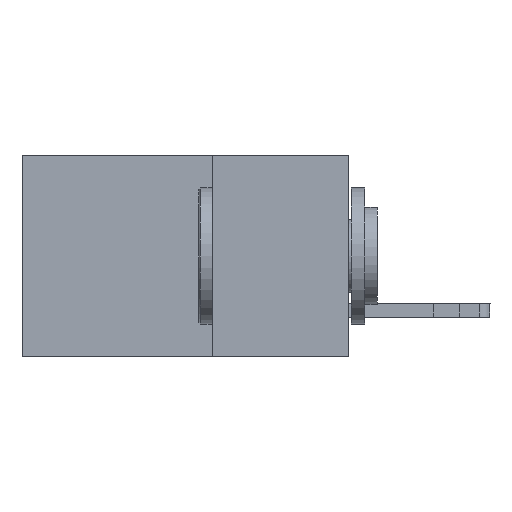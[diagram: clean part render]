
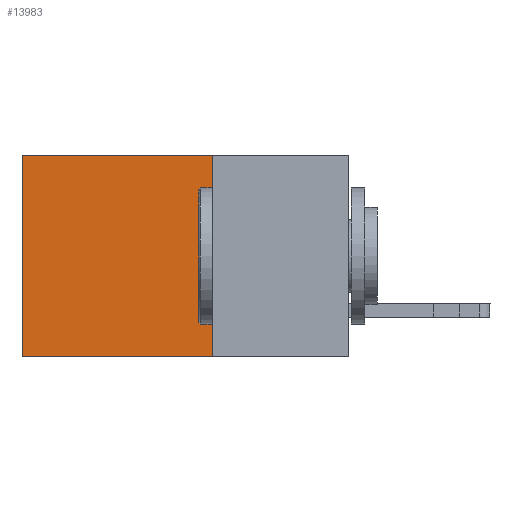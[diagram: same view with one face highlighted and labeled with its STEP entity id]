
A CAD part, left-side view. The second image highlights one B-rep face of the part: STEP entity #13983.
In plain terms, the highlighted planar face has unit normal (-1, 0, 0).
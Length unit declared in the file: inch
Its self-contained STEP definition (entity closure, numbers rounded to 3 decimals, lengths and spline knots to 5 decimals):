
#703 = LINE ( 'NONE', #4443, #17010 ) ;
#2767 = CARTESIAN_POINT ( 'NONE',  ( 0.2615, 0.6, -0.37 ) ) ;
#2885 = CARTESIAN_POINT ( 'NONE',  ( 0.2615, 0.25, 0. ) ) ;
#3759 = DIRECTION ( 'NONE',  ( 0., 0., -1. ) ) ;
#4016 = ORIENTED_EDGE ( 'NONE', *, *, #19403, .F. ) ;
#4443 = CARTESIAN_POINT ( 'NONE',  ( 0.2615, 0.25, -0.37 ) ) ;
#4503 = LINE ( 'NONE', #18357, #18527 ) ;
#5138 = VERTEX_POINT ( 'NONE', #12744 ) ;
#5658 = ORIENTED_EDGE ( 'NONE', *, *, #18680, .T. ) ;
#6020 = DIRECTION ( 'NONE',  ( 0., 1., 0. ) ) ;
#6075 = ORIENTED_EDGE ( 'NONE', *, *, #10573, .T. ) ;
#6719 = CARTESIAN_POINT ( 'NONE',  ( 0.2615, 0.25, -0.37 ) ) ;
#7590 = LINE ( 'NONE', #10888, #20680 ) ;
#8981 = AXIS2_PLACEMENT_3D ( 'NONE', #6719, #16838, #18879 ) ;
#9299 = ORIENTED_EDGE ( 'NONE', *, *, #15536, .F. ) ;
#9724 = DIRECTION ( 'NONE',  ( 0., 0., -1. ) ) ;
#10449 = VERTEX_POINT ( 'NONE', #2767 ) ;
#10477 = CARTESIAN_POINT ( 'NONE',  ( 0.2615, 0.25, -0.37 ) ) ;
#10573 = EDGE_CURVE ( 'NONE', #19845, #5138, #11386, .T. ) ;
#10888 = CARTESIAN_POINT ( 'NONE',  ( 0.2615, 0.6, -0.37 ) ) ;
#11386 = LINE ( 'NONE', #18652, #13593 ) ;
#11951 = DIRECTION ( 'NONE',  ( 0., 1., 0. ) ) ;
#12744 = CARTESIAN_POINT ( 'NONE',  ( 0.2615, 0.6, 0. ) ) ;
#13526 = FACE_OUTER_BOUND ( 'NONE', #14121, .T. ) ;
#13593 = VECTOR ( 'NONE', #11951, 39.37008 ) ;
#13983 = ADVANCED_FACE ( 'NONE', ( #13526 ), #20343, .F. ) ;
#14121 = EDGE_LOOP ( 'NONE', ( #5658, #9299, #4016, #6075 ) ) ;
#15373 = VERTEX_POINT ( 'NONE', #10477 ) ;
#15536 = EDGE_CURVE ( 'NONE', #15373, #10449, #703, .T. ) ;
#16838 = DIRECTION ( 'NONE',  ( 1., 0., 0. ) ) ;
#17010 = VECTOR ( 'NONE', #6020, 39.37008 ) ;
#18357 = CARTESIAN_POINT ( 'NONE',  ( 0.2615, 0.25, -0.37 ) ) ;
#18527 = VECTOR ( 'NONE', #9724, 39.37008 ) ;
#18652 = CARTESIAN_POINT ( 'NONE',  ( 0.2615, 0.25, 0. ) ) ;
#18680 = EDGE_CURVE ( 'NONE', #5138, #10449, #7590, .T. ) ;
#18879 = DIRECTION ( 'NONE',  ( 0., 0., -1. ) ) ;
#19403 = EDGE_CURVE ( 'NONE', #19845, #15373, #4503, .T. ) ;
#19845 = VERTEX_POINT ( 'NONE', #2885 ) ;
#20343 = PLANE ( 'NONE',  #8981 ) ;
#20680 = VECTOR ( 'NONE', #3759, 39.37008 ) ;
